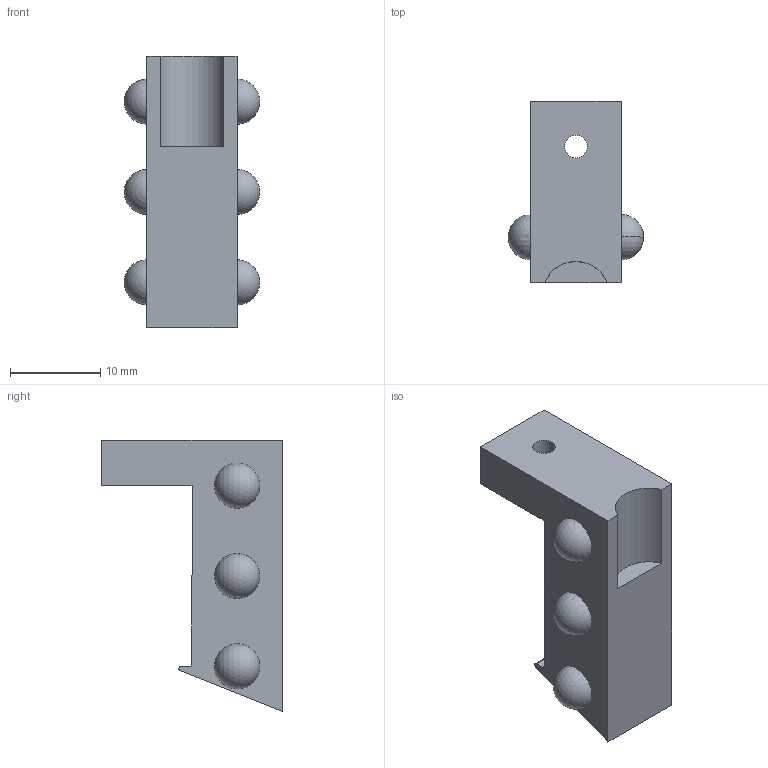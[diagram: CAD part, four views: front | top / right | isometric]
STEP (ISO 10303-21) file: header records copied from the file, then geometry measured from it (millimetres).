
FILE_DESCRIPTION (( 'STEP AP214' ), '1' );
FILE_NAME ('Bottom_Thumb_Tack_Holder.STEP', '2013-11-21T02:43:37', ( '' ), ( '' ), 'SwSTEP 2.0', 'SolidWorks 2013', '' );
FILE_SCHEMA (( 'AUTOMOTIVE_DESIGN' ));
Length unit declared in the file: millimetre
Products named in the file (1): Bottom_Thumb_Tack_Holder
Bounding box: 14.98 x 20 x 30 mm (x, y, z)
Volume: 3328.4 mm3; surface area: 1830 mm2
Topology: 1 solids, 1 shells, 32 faces, 95 edges, 60 vertices
Faces by surface type: plane 11, sphere 9, cylinder 8, torus 4
Entity records: 948 total; most frequent: DIRECTION 176, CARTESIAN_POINT 152, ORIENTED_EDGE 142, AXIS2_PLACEMENT_3D 72, EDGE_CURVE 71, VERTEX_POINT 48, EDGE_LOOP 41, CIRCLE 39
